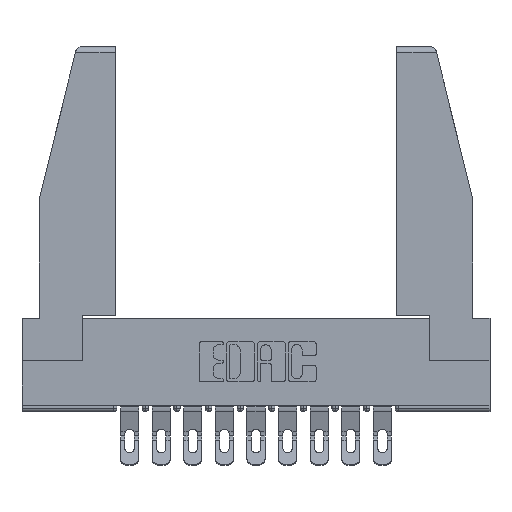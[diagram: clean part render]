
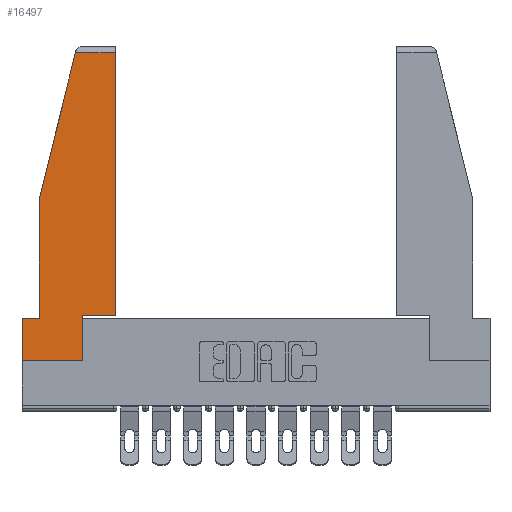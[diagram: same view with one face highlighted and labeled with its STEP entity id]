
A CAD part, top view. The second image highlights one B-rep face of the part: STEP entity #16497.
In plain terms, the highlighted planar face has unit normal (0, 0, 1).
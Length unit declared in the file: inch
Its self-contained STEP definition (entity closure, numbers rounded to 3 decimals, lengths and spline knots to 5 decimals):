
#93 = CARTESIAN_POINT ( 'NONE',  ( 0., 0., 0. ) ) ;
#180 = CARTESIAN_POINT ( 'NONE',  ( 0.086, 0.21, 0. ) ) ;
#1179 = VERTEX_POINT ( 'NONE', #8405 ) ;
#1435 = CARTESIAN_POINT ( 'NONE',  ( 0.461, 0.223, 0. ) ) ;
#1711 = DIRECTION ( 'NONE',  ( 0., -1., 0. ) ) ;
#1982 = VECTOR ( 'NONE', #15058, 39.37008 ) ;
#2133 = VECTOR ( 'NONE', #1711, 39.37008 ) ;
#2224 = CARTESIAN_POINT ( 'NONE',  ( 0.297, 0.223, 0. ) ) ;
#2457 = VECTOR ( 'NONE', #8779, 39.37008 ) ;
#2462 = VECTOR ( 'NONE', #14422, 39.37008 ) ;
#2613 = CARTESIAN_POINT ( 'NONE',  ( 0.297, 0., 0. ) ) ;
#3365 = ORIENTED_EDGE ( 'NONE', *, *, #4750, .T. ) ;
#3669 = VECTOR ( 'NONE', #5295, 39.37008 ) ;
#3723 = EDGE_CURVE ( 'NONE', #1179, #14913, #10806, .T. ) ;
#3766 = VERTEX_POINT ( 'NONE', #1435 ) ;
#3827 = CARTESIAN_POINT ( 'NONE',  ( 0.2636, 1.52, 0. ) ) ;
#4118 = LINE ( 'NONE', #2224, #11300 ) ;
#4150 = EDGE_CURVE ( 'NONE', #12958, #1179, #10789, .T. ) ;
#4430 = DIRECTION ( 'NONE',  ( 0., 1., 0. ) ) ;
#4486 = CARTESIAN_POINT ( 'NONE',  ( 0.297, 0., 0. ) ) ;
#4750 = EDGE_CURVE ( 'NONE', #11612, #3766, #4118, .T. ) ;
#4769 = ORIENTED_EDGE ( 'NONE', *, *, #8298, .T. ) ;
#5055 = CARTESIAN_POINT ( 'NONE',  ( 0., 1.52, 0. ) ) ;
#5256 = LINE ( 'NONE', #93, #3669 ) ;
#5295 = DIRECTION ( 'NONE',  ( 1., 0., 0. ) ) ;
#5443 = CARTESIAN_POINT ( 'NONE',  ( 0.086, 0.8, 0. ) ) ;
#5468 = ORIENTED_EDGE ( 'NONE', *, *, #3723, .T. ) ;
#5740 = ORIENTED_EDGE ( 'NONE', *, *, #7046, .T. ) ;
#6282 = ORIENTED_EDGE ( 'NONE', *, *, #4150, .T. ) ;
#6362 = CARTESIAN_POINT ( 'NONE',  ( 0.461, 1.52, 0. ) ) ;
#6469 = CARTESIAN_POINT ( 'NONE',  ( 0.271, 1.55, 0. ) ) ;
#6815 = VECTOR ( 'NONE', #7672, 39.37008 ) ;
#6933 = DIRECTION ( 'NONE',  ( -1., 0., 0. ) ) ;
#7046 = EDGE_CURVE ( 'NONE', #14913, #16828, #5256, .T. ) ;
#7239 = LINE ( 'NONE', #14856, #1982 ) ;
#7655 = CARTESIAN_POINT ( 'NONE',  ( 0.297, 0.223, 0. ) ) ;
#7672 = DIRECTION ( 'NONE',  ( -1., 0., 0. ) ) ;
#7988 = EDGE_LOOP ( 'NONE', ( #4769, #11227, #8444, #15877, #6282, #5468, #5740, #12507, #3365 ) ) ;
#8226 = LINE ( 'NONE', #5443, #2133 ) ;
#8298 = EDGE_CURVE ( 'NONE', #3766, #16562, #7239, .T. ) ;
#8405 = CARTESIAN_POINT ( 'NONE',  ( 0., 0.21, 0. ) ) ;
#8444 = ORIENTED_EDGE ( 'NONE', *, *, #15083, .T. ) ;
#8542 = CARTESIAN_POINT ( 'NONE',  ( 0., 0., 0. ) ) ;
#8779 = DIRECTION ( 'NONE',  ( 0., -1., 0. ) ) ;
#9185 = AXIS2_PLACEMENT_3D ( 'NONE', #11366, #12730, #11411 ) ;
#9968 = DIRECTION ( 'NONE',  ( 1., 0., 0. ) ) ;
#10264 = EDGE_CURVE ( 'NONE', #16828, #11612, #14552, .T. ) ;
#10627 = EDGE_CURVE ( 'NONE', #16412, #12958, #8226, .T. ) ;
#10789 = LINE ( 'NONE', #12013, #14465 ) ;
#10806 = LINE ( 'NONE', #14207, #2457 ) ;
#11076 = VECTOR ( 'NONE', #4430, 39.37008 ) ;
#11227 = ORIENTED_EDGE ( 'NONE', *, *, #11357, .T. ) ;
#11300 = VECTOR ( 'NONE', #9968, 39.37008 ) ;
#11357 = EDGE_CURVE ( 'NONE', #16562, #15121, #12767, .T. ) ;
#11366 = CARTESIAN_POINT ( 'NONE',  ( 0., 0., 0. ) ) ;
#11411 = DIRECTION ( 'NONE',  ( 1., 0., 0. ) ) ;
#11612 = VERTEX_POINT ( 'NONE', #7655 ) ;
#11630 = LINE ( 'NONE', #6469, #2462 ) ;
#12013 = CARTESIAN_POINT ( 'NONE',  ( 0., 0.21, 0. ) ) ;
#12507 = ORIENTED_EDGE ( 'NONE', *, *, #10264, .T. ) ;
#12730 = DIRECTION ( 'NONE',  ( 0., 0., 1. ) ) ;
#12767 = LINE ( 'NONE', #5055, #6815 ) ;
#12958 = VERTEX_POINT ( 'NONE', #180 ) ;
#14207 = CARTESIAN_POINT ( 'NONE',  ( 0., 0.21, 0. ) ) ;
#14243 = FACE_OUTER_BOUND ( 'NONE', #7988, .T. ) ;
#14422 = DIRECTION ( 'NONE',  ( -0.239, -0.971, 0. ) ) ;
#14465 = VECTOR ( 'NONE', #6933, 39.37008 ) ;
#14552 = LINE ( 'NONE', #4486, #11076 ) ;
#14856 = CARTESIAN_POINT ( 'NONE',  ( 0.461, 0.223, 0. ) ) ;
#14913 = VERTEX_POINT ( 'NONE', #8542 ) ;
#14944 = CARTESIAN_POINT ( 'NONE',  ( 0.086, 0.8, 0. ) ) ;
#15058 = DIRECTION ( 'NONE',  ( 0., 1., 0. ) ) ;
#15083 = EDGE_CURVE ( 'NONE', #15121, #16412, #11630, .T. ) ;
#15121 = VERTEX_POINT ( 'NONE', #3827 ) ;
#15877 = ORIENTED_EDGE ( 'NONE', *, *, #10627, .T. ) ;
#16412 = VERTEX_POINT ( 'NONE', #14944 ) ;
#16474 = PLANE ( 'NONE',  #9185 ) ;
#16497 = ADVANCED_FACE ( 'NONE', ( #14243 ), #16474, .T. ) ;
#16562 = VERTEX_POINT ( 'NONE', #6362 ) ;
#16828 = VERTEX_POINT ( 'NONE', #2613 ) ;
